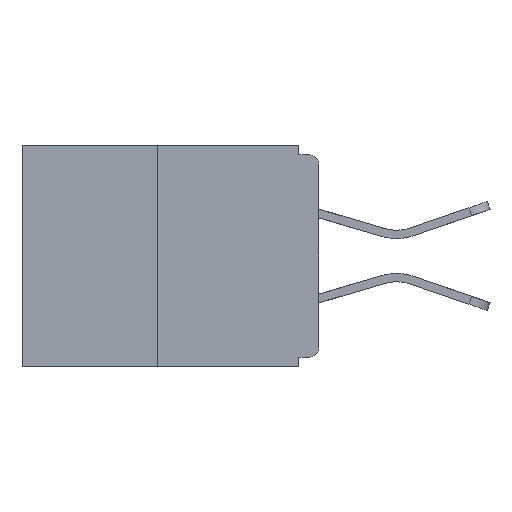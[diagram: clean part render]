
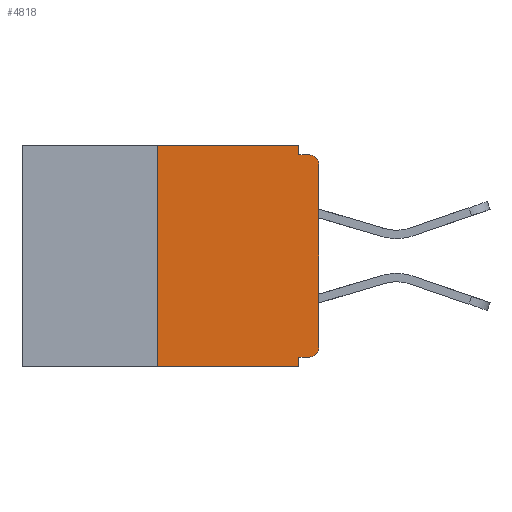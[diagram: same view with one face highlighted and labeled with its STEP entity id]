
A CAD part, left-side view. The second image highlights one B-rep face of the part: STEP entity #4818.
In plain terms, the highlighted planar face has unit normal (-1, 0, 0).
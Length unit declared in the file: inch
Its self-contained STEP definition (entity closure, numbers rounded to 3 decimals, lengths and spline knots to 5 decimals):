
#43 = LINE ( 'NONE', #13661, #17667 ) ;
#547 = LINE ( 'NONE', #13481, #6089 ) ;
#777 = VECTOR ( 'NONE', #4989, 39.37008 ) ;
#869 = EDGE_CURVE ( 'NONE', #17771, #1075, #1655, .T. ) ;
#872 = ORIENTED_EDGE ( 'NONE', *, *, #869, .F. ) ;
#973 = VERTEX_POINT ( 'NONE', #1124 ) ;
#986 = DIRECTION ( 'NONE',  ( 0., 0., -1. ) ) ;
#1051 = EDGE_LOOP ( 'NONE', ( #3000, #16136, #4682, #7728, #15438, #13299, #3566, #10414, #872, #11247 ) ) ;
#1075 = VERTEX_POINT ( 'NONE', #12889 ) ;
#1097 = VERTEX_POINT ( 'NONE', #17610 ) ;
#1124 = CARTESIAN_POINT ( 'NONE',  ( 0., 0.25, -0.343 ) ) ;
#1270 = LINE ( 'NONE', #12437, #9037 ) ;
#1425 = CIRCLE ( 'NONE', #7682, 0.015 ) ;
#1655 = LINE ( 'NONE', #3151, #2994 ) ;
#1719 = CARTESIAN_POINT ( 'NONE',  ( 0., 0.46, 0. ) ) ;
#1779 = DIRECTION ( 'NONE',  ( 0., 0., -1. ) ) ;
#2486 = EDGE_CURVE ( 'NONE', #11826, #9327, #5228, .T. ) ;
#2498 = EDGE_CURVE ( 'NONE', #973, #4277, #14494, .T. ) ;
#2519 = DIRECTION ( 'NONE',  ( 0., 0., 1. ) ) ;
#2994 = VECTOR ( 'NONE', #4774, 39.37008 ) ;
#3000 = ORIENTED_EDGE ( 'NONE', *, *, #3748, .F. ) ;
#3022 = EDGE_CURVE ( 'NONE', #1097, #1075, #1425, .T. ) ;
#3151 = CARTESIAN_POINT ( 'NONE',  ( 0., 0., -0.015 ) ) ;
#3566 = ORIENTED_EDGE ( 'NONE', *, *, #14029, .T. ) ;
#3748 = EDGE_CURVE ( 'NONE', #4277, #4687, #4522, .T. ) ;
#4277 = VERTEX_POINT ( 'NONE', #10658 ) ;
#4510 = CARTESIAN_POINT ( 'NONE',  ( 0., 0., -0.328 ) ) ;
#4522 = LINE ( 'NONE', #5213, #16410 ) ;
#4576 = DIRECTION ( 'NONE',  ( 1., 0., 0. ) ) ;
#4682 = ORIENTED_EDGE ( 'NONE', *, *, #17497, .T. ) ;
#4687 = VERTEX_POINT ( 'NONE', #14138 ) ;
#4774 = DIRECTION ( 'NONE',  ( 0., -1., 0. ) ) ;
#4818 = ADVANCED_FACE ( 'NONE', ( #11793 ), #10284, .F. ) ;
#4887 = DIRECTION ( 'NONE',  ( 0., 0., -1. ) ) ;
#4989 = DIRECTION ( 'NONE',  ( 0., 0., -1. ) ) ;
#5048 = DIRECTION ( 'NONE',  ( 0., 0., 1. ) ) ;
#5213 = CARTESIAN_POINT ( 'NONE',  ( 0., 0.46, 0. ) ) ;
#5228 = LINE ( 'NONE', #17547, #777 ) ;
#6089 = VECTOR ( 'NONE', #17588, 39.37008 ) ;
#6918 = VERTEX_POINT ( 'NONE', #14762 ) ;
#7328 = AXIS2_PLACEMENT_3D ( 'NONE', #1719, #4576, #1779 ) ;
#7682 = AXIS2_PLACEMENT_3D ( 'NONE', #10581, #17510, #4887 ) ;
#7728 = ORIENTED_EDGE ( 'NONE', *, *, #2486, .F. ) ;
#9037 = VECTOR ( 'NONE', #13797, 39.37008 ) ;
#9327 = VERTEX_POINT ( 'NONE', #14342 ) ;
#10035 = CARTESIAN_POINT ( 'NONE',  ( 0., 0., -0.313 ) ) ;
#10284 = PLANE ( 'NONE',  #7328 ) ;
#10414 = ORIENTED_EDGE ( 'NONE', *, *, #3022, .T. ) ;
#10581 = CARTESIAN_POINT ( 'NONE',  ( 0., 0.015, -0.03 ) ) ;
#10658 = CARTESIAN_POINT ( 'NONE',  ( 0., 0.25, 0. ) ) ;
#11247 = ORIENTED_EDGE ( 'NONE', *, *, #12043, .F. ) ;
#11402 = VECTOR ( 'NONE', #5048, 39.37008 ) ;
#11487 = VECTOR ( 'NONE', #17185, 39.37008 ) ;
#11749 = CIRCLE ( 'NONE', #15717, 0.015 ) ;
#11793 = FACE_OUTER_BOUND ( 'NONE', #1051, .T. ) ;
#11826 = VERTEX_POINT ( 'NONE', #13413 ) ;
#12043 = EDGE_CURVE ( 'NONE', #4687, #17771, #547, .T. ) ;
#12319 = CARTESIAN_POINT ( 'NONE',  ( 0., 0.015, -0.313 ) ) ;
#12437 = CARTESIAN_POINT ( 'NONE',  ( 0., 0.46, -0.343 ) ) ;
#12831 = LINE ( 'NONE', #4510, #11487 ) ;
#12889 = CARTESIAN_POINT ( 'NONE',  ( 0., 0.015, -0.015 ) ) ;
#13299 = ORIENTED_EDGE ( 'NONE', *, *, #14447, .T. ) ;
#13390 = CARTESIAN_POINT ( 'NONE',  ( 0., 0.25, 0. ) ) ;
#13413 = CARTESIAN_POINT ( 'NONE',  ( 0., 0.031, -0.328 ) ) ;
#13481 = CARTESIAN_POINT ( 'NONE',  ( 0., 0.031, 0. ) ) ;
#13488 = DIRECTION ( 'NONE',  ( 0., -1., 0. ) ) ;
#13661 = CARTESIAN_POINT ( 'NONE',  ( 0., 0., 0. ) ) ;
#13731 = DIRECTION ( 'NONE',  ( -1., 0., 0. ) ) ;
#13797 = DIRECTION ( 'NONE',  ( 0., -1., 0. ) ) ;
#14029 = EDGE_CURVE ( 'NONE', #17190, #1097, #43, .T. ) ;
#14138 = CARTESIAN_POINT ( 'NONE',  ( 0., 0.031, 0. ) ) ;
#14342 = CARTESIAN_POINT ( 'NONE',  ( 0., 0.031, -0.343 ) ) ;
#14447 = EDGE_CURVE ( 'NONE', #6918, #17190, #11749, .T. ) ;
#14494 = LINE ( 'NONE', #13390, #11402 ) ;
#14762 = CARTESIAN_POINT ( 'NONE',  ( 0., 0.015, -0.328 ) ) ;
#15438 = ORIENTED_EDGE ( 'NONE', *, *, #16839, .F. ) ;
#15717 = AXIS2_PLACEMENT_3D ( 'NONE', #12319, #13731, #986 ) ;
#16136 = ORIENTED_EDGE ( 'NONE', *, *, #2498, .F. ) ;
#16368 = CARTESIAN_POINT ( 'NONE',  ( 0., 0.031, -0.015 ) ) ;
#16410 = VECTOR ( 'NONE', #13488, 39.37008 ) ;
#16839 = EDGE_CURVE ( 'NONE', #6918, #11826, #12831, .T. ) ;
#17185 = DIRECTION ( 'NONE',  ( 0., 1., 0. ) ) ;
#17190 = VERTEX_POINT ( 'NONE', #10035 ) ;
#17497 = EDGE_CURVE ( 'NONE', #973, #9327, #1270, .T. ) ;
#17510 = DIRECTION ( 'NONE',  ( -1., 0., 0. ) ) ;
#17547 = CARTESIAN_POINT ( 'NONE',  ( 0., 0.031, -0.343 ) ) ;
#17588 = DIRECTION ( 'NONE',  ( 0., 0., -1. ) ) ;
#17610 = CARTESIAN_POINT ( 'NONE',  ( 0., 0., -0.03 ) ) ;
#17667 = VECTOR ( 'NONE', #2519, 39.37008 ) ;
#17771 = VERTEX_POINT ( 'NONE', #16368 ) ;
